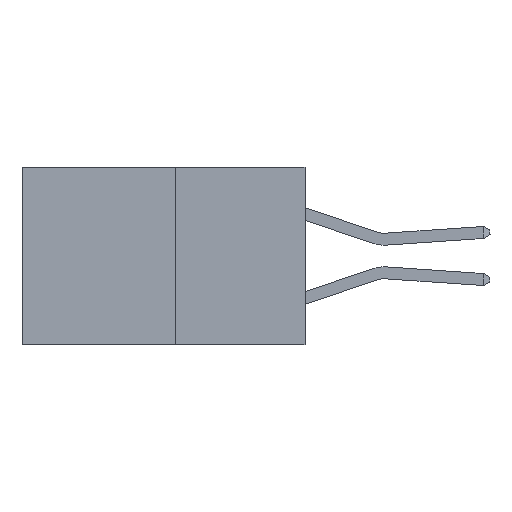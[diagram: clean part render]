
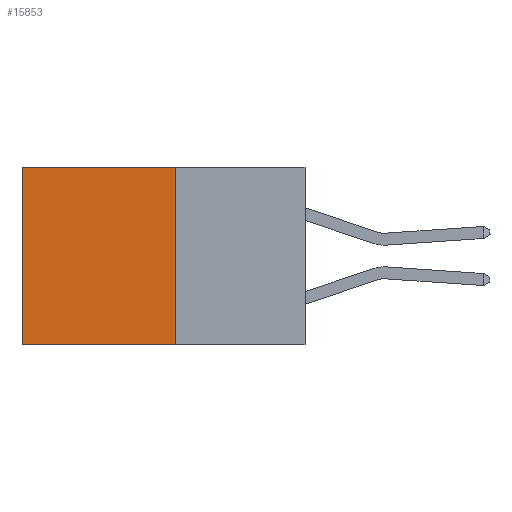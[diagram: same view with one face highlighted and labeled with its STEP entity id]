
A CAD part, left-side view. The second image highlights one B-rep face of the part: STEP entity #15853.
In plain terms, the highlighted planar face has unit normal (-1, 0, 0).
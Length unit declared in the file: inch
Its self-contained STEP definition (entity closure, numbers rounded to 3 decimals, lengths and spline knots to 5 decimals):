
#781 = DIRECTION ( 'NONE',  ( 0., 0., -1. ) ) ;
#1238 = VERTEX_POINT ( 'NONE', #14331 ) ;
#1574 = EDGE_CURVE ( 'NONE', #1588, #4340, #13602, .T. ) ;
#1588 = VERTEX_POINT ( 'NONE', #3783 ) ;
#1608 = CARTESIAN_POINT ( 'NONE',  ( 0.277, 0.27, -0.37 ) ) ;
#1791 = AXIS2_PLACEMENT_3D ( 'NONE', #4043, #10964, #781 ) ;
#2075 = VECTOR ( 'NONE', #2310, 39.37008 ) ;
#2310 = DIRECTION ( 'NONE',  ( 0., 0., -1. ) ) ;
#2577 = LINE ( 'NONE', #1608, #6640 ) ;
#3274 = EDGE_CURVE ( 'NONE', #1588, #9069, #6662, .T. ) ;
#3659 = CARTESIAN_POINT ( 'NONE',  ( 0.277, 0.27, 0. ) ) ;
#3783 = CARTESIAN_POINT ( 'NONE',  ( 0.277, 0.27, 0. ) ) ;
#4043 = CARTESIAN_POINT ( 'NONE',  ( 0.277, 0.27, -0.37 ) ) ;
#4340 = VERTEX_POINT ( 'NONE', #7658 ) ;
#4421 = DIRECTION ( 'NONE',  ( 0., 1., 0. ) ) ;
#5107 = VECTOR ( 'NONE', #4421, 39.37008 ) ;
#5521 = CARTESIAN_POINT ( 'NONE',  ( 0.277, 0.59, -0.37 ) ) ;
#6513 = LINE ( 'NONE', #5521, #14951 ) ;
#6640 = VECTOR ( 'NONE', #6814, 39.37008 ) ;
#6662 = LINE ( 'NONE', #9414, #2075 ) ;
#6814 = DIRECTION ( 'NONE',  ( 0., 1., 0. ) ) ;
#7658 = CARTESIAN_POINT ( 'NONE',  ( 0.277, 0.59, 0. ) ) ;
#8335 = ORIENTED_EDGE ( 'NONE', *, *, #3274, .F. ) ;
#8510 = EDGE_CURVE ( 'NONE', #4340, #1238, #6513, .T. ) ;
#9069 = VERTEX_POINT ( 'NONE', #13804 ) ;
#9414 = CARTESIAN_POINT ( 'NONE',  ( 0.277, 0.27, -0.37 ) ) ;
#9667 = ORIENTED_EDGE ( 'NONE', *, *, #17666, .F. ) ;
#9686 = ORIENTED_EDGE ( 'NONE', *, *, #1574, .T. ) ;
#10964 = DIRECTION ( 'NONE',  ( 1., 0., 0. ) ) ;
#11775 = FACE_OUTER_BOUND ( 'NONE', #15310, .T. ) ;
#13602 = LINE ( 'NONE', #3659, #5107 ) ;
#13804 = CARTESIAN_POINT ( 'NONE',  ( 0.277, 0.27, -0.37 ) ) ;
#13971 = DIRECTION ( 'NONE',  ( 0., 0., -1. ) ) ;
#14331 = CARTESIAN_POINT ( 'NONE',  ( 0.277, 0.59, -0.37 ) ) ;
#14951 = VECTOR ( 'NONE', #13971, 39.37008 ) ;
#15310 = EDGE_LOOP ( 'NONE', ( #19219, #9667, #8335, #9686 ) ) ;
#15853 = ADVANCED_FACE ( 'NONE', ( #11775 ), #20746, .F. ) ;
#17666 = EDGE_CURVE ( 'NONE', #9069, #1238, #2577, .T. ) ;
#19219 = ORIENTED_EDGE ( 'NONE', *, *, #8510, .T. ) ;
#20746 = PLANE ( 'NONE',  #1791 ) ;
